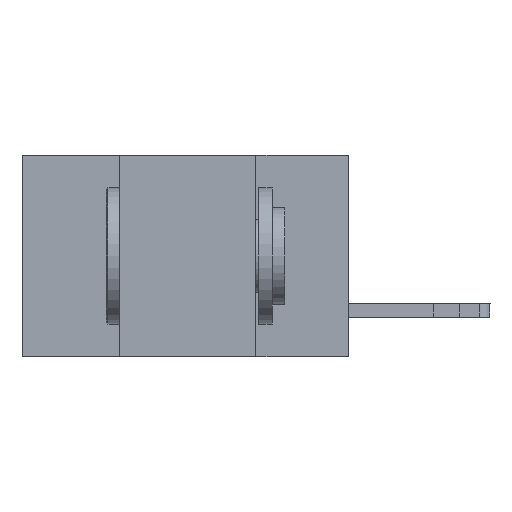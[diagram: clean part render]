
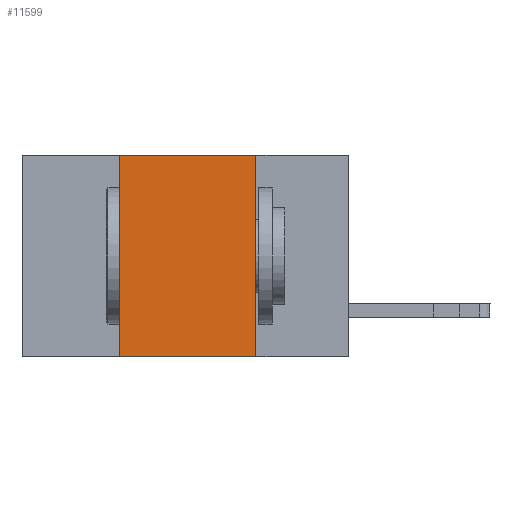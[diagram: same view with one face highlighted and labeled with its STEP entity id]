
A CAD part, left-side view. The second image highlights one B-rep face of the part: STEP entity #11599.
In plain terms, the highlighted planar face has unit normal (-1, 0, 0).
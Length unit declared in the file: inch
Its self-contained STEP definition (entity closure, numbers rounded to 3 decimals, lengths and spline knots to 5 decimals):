
#842 = CARTESIAN_POINT ( 'NONE',  ( 0., 0.17, -0.37 ) ) ;
#910 = EDGE_CURVE ( 'NONE', #13076, #4485, #2826, .T. ) ;
#1076 = VECTOR ( 'NONE', #10268, 39.37008 ) ;
#1226 = DIRECTION ( 'NONE',  ( 0., -1., 0. ) ) ;
#1730 = DIRECTION ( 'NONE',  ( 0., 0., -1. ) ) ;
#2826 = LINE ( 'NONE', #842, #8397 ) ;
#2884 = CARTESIAN_POINT ( 'NONE',  ( 0., 0.6, -0.37 ) ) ;
#3582 = EDGE_CURVE ( 'NONE', #5893, #13076, #8351, .T. ) ;
#4485 = VERTEX_POINT ( 'NONE', #8705 ) ;
#4652 = EDGE_CURVE ( 'NONE', #10004, #4485, #8094, .T. ) ;
#4768 = CARTESIAN_POINT ( 'NONE',  ( 0., 0.42, -0.37 ) ) ;
#5121 = ORIENTED_EDGE ( 'NONE', *, *, #4652, .T. ) ;
#5893 = VERTEX_POINT ( 'NONE', #10003 ) ;
#5965 = CARTESIAN_POINT ( 'NONE',  ( 0., 0.17, 0. ) ) ;
#6182 = CARTESIAN_POINT ( 'NONE',  ( 0., 0.6, 0. ) ) ;
#6271 = CARTESIAN_POINT ( 'NONE',  ( 0., 0.42, -0.37 ) ) ;
#6653 = DIRECTION ( 'NONE',  ( 0., 0., -1. ) ) ;
#7082 = CARTESIAN_POINT ( 'NONE',  ( 0., 0.6, 0. ) ) ;
#7562 = EDGE_CURVE ( 'NONE', #10004, #5893, #9390, .T. ) ;
#8094 = LINE ( 'NONE', #2884, #1076 ) ;
#8100 = FACE_OUTER_BOUND ( 'NONE', #8690, .T. ) ;
#8232 = PLANE ( 'NONE',  #10281 ) ;
#8305 = ORIENTED_EDGE ( 'NONE', *, *, #3582, .F. ) ;
#8351 = LINE ( 'NONE', #6182, #13393 ) ;
#8387 = ORIENTED_EDGE ( 'NONE', *, *, #910, .F. ) ;
#8397 = VECTOR ( 'NONE', #1730, 39.37008 ) ;
#8690 = EDGE_LOOP ( 'NONE', ( #8387, #8305, #9906, #5121 ) ) ;
#8705 = CARTESIAN_POINT ( 'NONE',  ( 0., 0.17, -0.37 ) ) ;
#9390 = LINE ( 'NONE', #6271, #10235 ) ;
#9906 = ORIENTED_EDGE ( 'NONE', *, *, #7562, .F. ) ;
#10003 = CARTESIAN_POINT ( 'NONE',  ( 0., 0.42, 0. ) ) ;
#10004 = VERTEX_POINT ( 'NONE', #4768 ) ;
#10145 = DIRECTION ( 'NONE',  ( 0., 0., 1. ) ) ;
#10235 = VECTOR ( 'NONE', #10145, 39.37008 ) ;
#10268 = DIRECTION ( 'NONE',  ( 0., -1., 0. ) ) ;
#10281 = AXIS2_PLACEMENT_3D ( 'NONE', #7082, #11216, #6653 ) ;
#11216 = DIRECTION ( 'NONE',  ( 1., 0., 0. ) ) ;
#11599 = ADVANCED_FACE ( 'NONE', ( #8100 ), #8232, .F. ) ;
#13076 = VERTEX_POINT ( 'NONE', #5965 ) ;
#13393 = VECTOR ( 'NONE', #1226, 39.37008 ) ;
